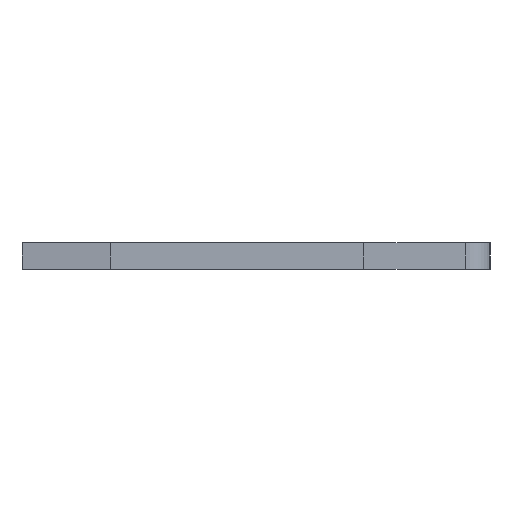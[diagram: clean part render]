
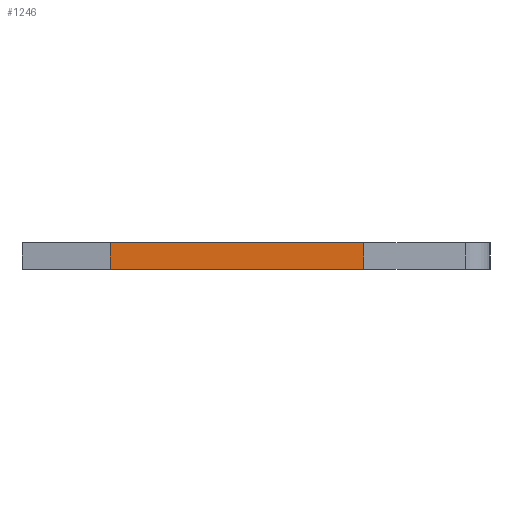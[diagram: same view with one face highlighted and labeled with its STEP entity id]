
A CAD part, left-side view. The second image highlights one B-rep face of the part: STEP entity #1246.
In plain terms, the highlighted face is planar.
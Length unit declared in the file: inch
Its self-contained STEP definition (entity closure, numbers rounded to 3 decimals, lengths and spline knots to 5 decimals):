
#25 = CARTESIAN_POINT ( 'NONE',  ( -0.013, 0.146, -0.0575 ) ) ;
#38 = VECTOR ( 'NONE', #1237, 39.37008 ) ;
#91 = LINE ( 'NONE', #473, #38 ) ;
#141 = DIRECTION ( 'NONE',  ( 0., 1., 0. ) ) ;
#144 = CARTESIAN_POINT ( 'NONE',  ( -0.013, 0.146, -0.0575 ) ) ;
#168 = VECTOR ( 'NONE', #733, 39.37008 ) ;
#235 = DIRECTION ( 'NONE',  ( 0., 0., 1. ) ) ;
#249 = AXIS2_PLACEMENT_3D ( 'NONE', #1312, #235, #1068 ) ;
#257 = CARTESIAN_POINT ( 'NONE',  ( 0.013, 0.146, -0.0575 ) ) ;
#337 = VECTOR ( 'NONE', #551, 39.37008 ) ;
#405 = EDGE_LOOP ( 'NONE', ( #752, #1091, #497, #468 ) ) ;
#450 = VECTOR ( 'NONE', #141, 39.37008 ) ;
#468 = ORIENTED_EDGE ( 'NONE', *, *, #1514, .T. ) ;
#473 = CARTESIAN_POINT ( 'NONE',  ( 0.013, -0.099, -0.0575 ) ) ;
#497 = ORIENTED_EDGE ( 'NONE', *, *, #775, .F. ) ;
#548 = CARTESIAN_POINT ( 'NONE',  ( -0.013, -0.099, -0.0575 ) ) ;
#551 = DIRECTION ( 'NONE',  ( -1., 0., 0. ) ) ;
#561 = CARTESIAN_POINT ( 'NONE',  ( 0.013, 0.146, -0.0575 ) ) ;
#612 = VERTEX_POINT ( 'NONE', #1453 ) ;
#722 = CARTESIAN_POINT ( 'NONE',  ( 0.013, -0.099, -0.0575 ) ) ;
#733 = DIRECTION ( 'NONE',  ( 0., 1., 0. ) ) ;
#752 = ORIENTED_EDGE ( 'NONE', *, *, #880, .T. ) ;
#769 = VERTEX_POINT ( 'NONE', #722 ) ;
#775 = EDGE_CURVE ( 'NONE', #769, #612, #777, .T. ) ;
#777 = LINE ( 'NONE', #257, #168 ) ;
#834 = PLANE ( 'NONE',  #249 ) ;
#880 = EDGE_CURVE ( 'NONE', #1062, #940, #1096, .T. ) ;
#940 = VERTEX_POINT ( 'NONE', #25 ) ;
#958 = EDGE_CURVE ( 'NONE', #612, #940, #1534, .T. ) ;
#1062 = VERTEX_POINT ( 'NONE', #548 ) ;
#1068 = DIRECTION ( 'NONE',  ( 1., 0., 0. ) ) ;
#1091 = ORIENTED_EDGE ( 'NONE', *, *, #958, .F. ) ;
#1096 = LINE ( 'NONE', #144, #450 ) ;
#1237 = DIRECTION ( 'NONE',  ( -1., 0., 0. ) ) ;
#1246 = ADVANCED_FACE ( 'NONE', ( #1516 ), #834, .F. ) ;
#1312 = CARTESIAN_POINT ( 'NONE',  ( 0.013, 0.146, -0.0575 ) ) ;
#1453 = CARTESIAN_POINT ( 'NONE',  ( 0.013, 0.146, -0.0575 ) ) ;
#1514 = EDGE_CURVE ( 'NONE', #769, #1062, #91, .T. ) ;
#1516 = FACE_OUTER_BOUND ( 'NONE', #405, .T. ) ;
#1534 = LINE ( 'NONE', #561, #337 ) ;
